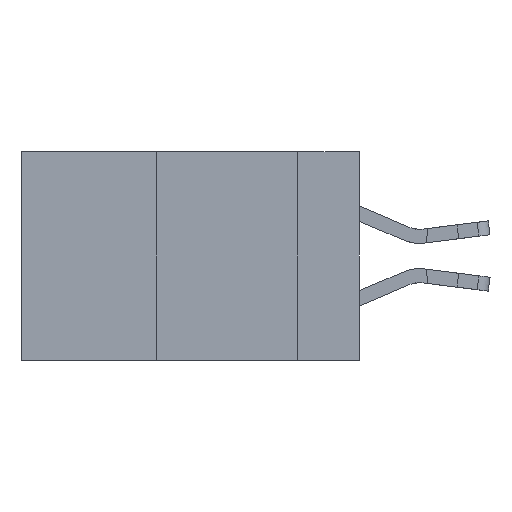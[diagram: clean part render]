
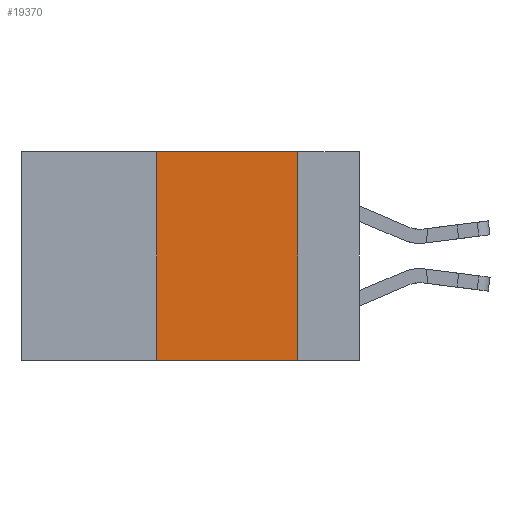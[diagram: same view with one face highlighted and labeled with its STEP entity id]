
A CAD part, left-side view. The second image highlights one B-rep face of the part: STEP entity #19370.
In plain terms, the highlighted planar face has unit normal (-1, 0, 0).
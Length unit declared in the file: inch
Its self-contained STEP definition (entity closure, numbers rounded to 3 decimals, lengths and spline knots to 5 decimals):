
#258 = AXIS2_PLACEMENT_3D ( 'NONE', #14765, #14683, #2201 ) ;
#1259 = VECTOR ( 'NONE', #6207, 39.37008 ) ;
#2097 = EDGE_CURVE ( 'NONE', #12596, #27200, #5666, .T. ) ;
#2201 = DIRECTION ( 'NONE',  ( 0., 0., -1. ) ) ;
#2468 = CARTESIAN_POINT ( 'NONE',  ( 0., 0.36, 0. ) ) ;
#2657 = ORIENTED_EDGE ( 'NONE', *, *, #19621, .F. ) ;
#3102 = ORIENTED_EDGE ( 'NONE', *, *, #2097, .F. ) ;
#3465 = EDGE_LOOP ( 'NONE', ( #3102, #7893, #2657, #7205 ) ) ;
#5666 = LINE ( 'NONE', #16232, #16245 ) ;
#5835 = DIRECTION ( 'NONE',  ( 0., -1., 0. ) ) ;
#6207 = DIRECTION ( 'NONE',  ( 0., -1., 0. ) ) ;
#6883 = LINE ( 'NONE', #25160, #1259 ) ;
#7205 = ORIENTED_EDGE ( 'NONE', *, *, #8560, .T. ) ;
#7473 = VECTOR ( 'NONE', #5835, 39.37008 ) ;
#7893 = ORIENTED_EDGE ( 'NONE', *, *, #16256, .F. ) ;
#8560 = EDGE_CURVE ( 'NONE', #15355, #27200, #6883, .T. ) ;
#9576 = DIRECTION ( 'NONE',  ( 0., 0., -1. ) ) ;
#11783 = LINE ( 'NONE', #27143, #7473 ) ;
#12596 = VERTEX_POINT ( 'NONE', #16242 ) ;
#13289 = VECTOR ( 'NONE', #21404, 39.37008 ) ;
#14683 = DIRECTION ( 'NONE',  ( 1., 0., 0. ) ) ;
#14765 = CARTESIAN_POINT ( 'NONE',  ( 0., 0.6, 0. ) ) ;
#15355 = VERTEX_POINT ( 'NONE', #17916 ) ;
#16232 = CARTESIAN_POINT ( 'NONE',  ( 0., 0.11, 0. ) ) ;
#16238 = LINE ( 'NONE', #2468, #13289 ) ;
#16242 = CARTESIAN_POINT ( 'NONE',  ( 0., 0.11, 0. ) ) ;
#16245 = VECTOR ( 'NONE', #9576, 39.37008 ) ;
#16256 = EDGE_CURVE ( 'NONE', #19580, #12596, #11783, .T. ) ;
#17916 = CARTESIAN_POINT ( 'NONE',  ( 0., 0.36, -0.37 ) ) ;
#18568 = CARTESIAN_POINT ( 'NONE',  ( 0., 0.11, -0.37 ) ) ;
#19116 = PLANE ( 'NONE',  #258 ) ;
#19370 = ADVANCED_FACE ( 'NONE', ( #23201 ), #19116, .F. ) ;
#19580 = VERTEX_POINT ( 'NONE', #23721 ) ;
#19621 = EDGE_CURVE ( 'NONE', #15355, #19580, #16238, .T. ) ;
#21404 = DIRECTION ( 'NONE',  ( 0., 0., 1. ) ) ;
#23201 = FACE_OUTER_BOUND ( 'NONE', #3465, .T. ) ;
#23721 = CARTESIAN_POINT ( 'NONE',  ( 0., 0.36, 0. ) ) ;
#25160 = CARTESIAN_POINT ( 'NONE',  ( 0., 0.6, -0.37 ) ) ;
#27143 = CARTESIAN_POINT ( 'NONE',  ( 0., 0.6, 0. ) ) ;
#27200 = VERTEX_POINT ( 'NONE', #18568 ) ;
